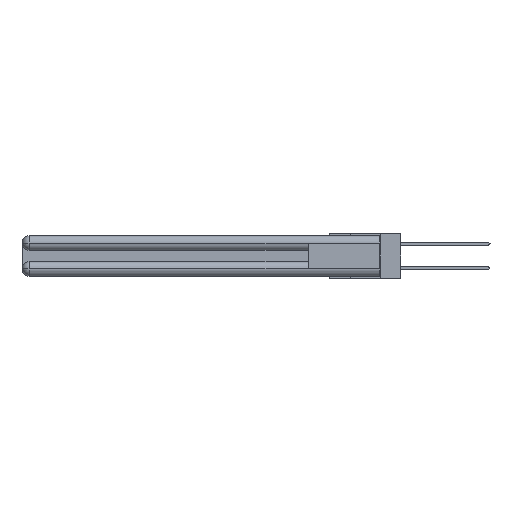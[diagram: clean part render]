
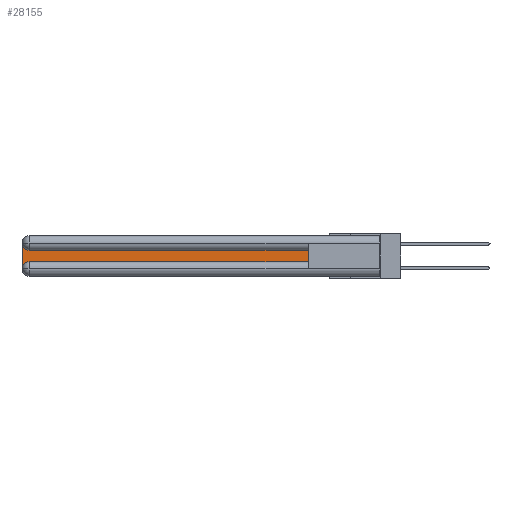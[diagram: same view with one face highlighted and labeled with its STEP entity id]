
A CAD part, left-side view. The second image highlights one B-rep face of the part: STEP entity #28155.
In plain terms, the highlighted planar face has unit normal (-1, 0, 0).
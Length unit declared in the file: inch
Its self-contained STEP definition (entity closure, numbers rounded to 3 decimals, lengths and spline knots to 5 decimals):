
#190 = PLANE ( 'NONE',  #26287 ) ;
#938 = CARTESIAN_POINT ( 'NONE',  ( 0.075, 3., -0.2775 ) ) ;
#1373 = CARTESIAN_POINT ( 'NONE',  ( 0.075, 2.94, -0.0625 ) ) ;
#1838 = ORIENTED_EDGE ( 'NONE', *, *, #20933, .T. ) ;
#2170 = CARTESIAN_POINT ( 'NONE',  ( 0.075, 0.6, -0.2175 ) ) ;
#2658 = VECTOR ( 'NONE', #31526, 39.37008 ) ;
#2902 = DIRECTION ( 'NONE',  ( 0., 0., -1. ) ) ;
#3857 = VERTEX_POINT ( 'NONE', #19541 ) ;
#4564 = VERTEX_POINT ( 'NONE', #938 ) ;
#5586 = DIRECTION ( 'NONE',  ( 0., 0., -1. ) ) ;
#6574 = DIRECTION ( 'NONE',  ( 1., 0., 0. ) ) ;
#6643 = LINE ( 'NONE', #26916, #22002 ) ;
#7579 = FACE_OUTER_BOUND ( 'NONE', #10476, .T. ) ;
#8238 = EDGE_CURVE ( 'NONE', #4564, #17016, #9254, .T. ) ;
#8392 = CARTESIAN_POINT ( 'NONE',  ( 0.075, 2.94, -0.2175 ) ) ;
#8486 = DIRECTION ( 'NONE',  ( 0., 0., -1. ) ) ;
#9254 = CIRCLE ( 'NONE', #20056, 0.06 ) ;
#9724 = EDGE_CURVE ( 'NONE', #17016, #3857, #6643, .T. ) ;
#10476 = EDGE_LOOP ( 'NONE', ( #19161, #31717, #1838, #29018, #19208, #12059 ) ) ;
#10626 = CARTESIAN_POINT ( 'NONE',  ( 0.075, 3., -0.1225 ) ) ;
#10731 = LINE ( 'NONE', #15659, #22762 ) ;
#11016 = AXIS2_PLACEMENT_3D ( 'NONE', #1373, #6574, #14300 ) ;
#12059 = ORIENTED_EDGE ( 'NONE', *, *, #18741, .T. ) ;
#12226 = DIRECTION ( 'NONE',  ( 0., 0., 1. ) ) ;
#13433 = CARTESIAN_POINT ( 'NONE',  ( 0.075, 2.94, -0.1225 ) ) ;
#13495 = CARTESIAN_POINT ( 'NONE',  ( 0.075, 0.6, -0.1225 ) ) ;
#14300 = DIRECTION ( 'NONE',  ( 0., 0., -1. ) ) ;
#15571 = DIRECTION ( 'NONE',  ( 1., 0., 0. ) ) ;
#15659 = CARTESIAN_POINT ( 'NONE',  ( 0.075, 3., -0.2175 ) ) ;
#16708 = VERTEX_POINT ( 'NONE', #30068 ) ;
#16729 = EDGE_CURVE ( 'NONE', #25628, #16708, #32456, .T. ) ;
#16870 = VECTOR ( 'NONE', #12226, 39.37008 ) ;
#17016 = VERTEX_POINT ( 'NONE', #8392 ) ;
#18741 = EDGE_CURVE ( 'NONE', #3857, #32041, #22927, .T. ) ;
#19161 = ORIENTED_EDGE ( 'NONE', *, *, #29046, .T. ) ;
#19208 = ORIENTED_EDGE ( 'NONE', *, *, #9724, .T. ) ;
#19541 = CARTESIAN_POINT ( 'NONE',  ( 0.075, 0.6, -0.2175 ) ) ;
#20056 = AXIS2_PLACEMENT_3D ( 'NONE', #29440, #23912, #8486 ) ;
#20933 = EDGE_CURVE ( 'NONE', #16708, #4564, #10731, .T. ) ;
#21623 = DIRECTION ( 'NONE',  ( 0., -1., 0. ) ) ;
#22002 = VECTOR ( 'NONE', #21623, 39.37008 ) ;
#22762 = VECTOR ( 'NONE', #5586, 39.37008 ) ;
#22927 = LINE ( 'NONE', #2170, #16870 ) ;
#23912 = DIRECTION ( 'NONE',  ( 1., 0., 0. ) ) ;
#25628 = VERTEX_POINT ( 'NONE', #13433 ) ;
#26287 = AXIS2_PLACEMENT_3D ( 'NONE', #10626, #15571, #2902 ) ;
#26866 = LINE ( 'NONE', #13495, #2658 ) ;
#26916 = CARTESIAN_POINT ( 'NONE',  ( 0.075, 0.6, -0.2175 ) ) ;
#28155 = ADVANCED_FACE ( 'NONE', ( #7579 ), #190, .F. ) ;
#29018 = ORIENTED_EDGE ( 'NONE', *, *, #8238, .T. ) ;
#29046 = EDGE_CURVE ( 'NONE', #32041, #25628, #26866, .T. ) ;
#29440 = CARTESIAN_POINT ( 'NONE',  ( 0.075, 2.94, -0.2775 ) ) ;
#30068 = CARTESIAN_POINT ( 'NONE',  ( 0.075, 3., -0.0625 ) ) ;
#30309 = CARTESIAN_POINT ( 'NONE',  ( 0.075, 0.6, -0.1225 ) ) ;
#31526 = DIRECTION ( 'NONE',  ( 0., 1., 0. ) ) ;
#31717 = ORIENTED_EDGE ( 'NONE', *, *, #16729, .T. ) ;
#32041 = VERTEX_POINT ( 'NONE', #30309 ) ;
#32456 = CIRCLE ( 'NONE', #11016, 0.06 ) ;
